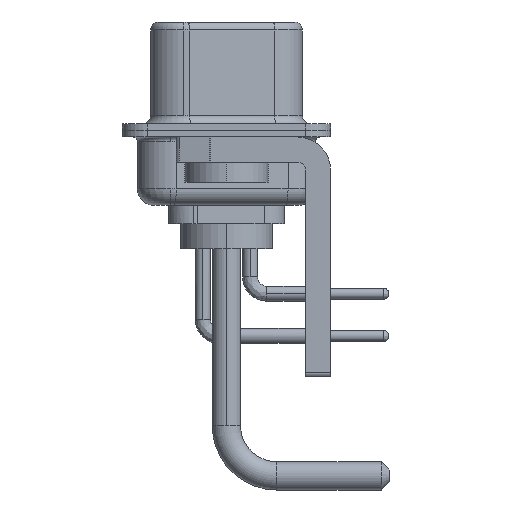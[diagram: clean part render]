
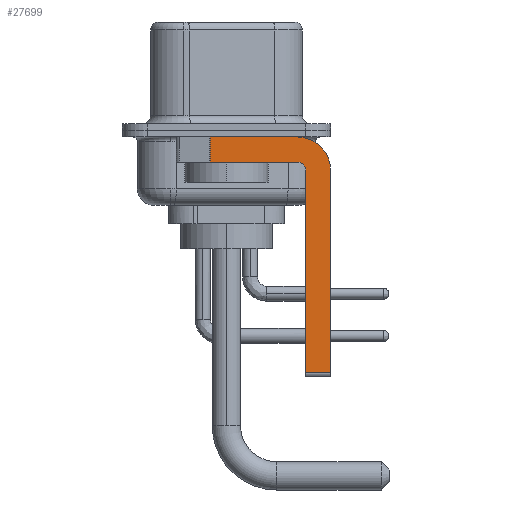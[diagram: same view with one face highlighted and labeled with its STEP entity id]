
A CAD part, left-side view. The second image highlights one B-rep face of the part: STEP entity #27699.
In plain terms, the highlighted planar face has unit normal (-1, 0, 0).
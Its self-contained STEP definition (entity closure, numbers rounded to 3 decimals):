
#1863 = VERTEX_POINT ( 'NONE', #11196 ) ;
#2065 = ORIENTED_EDGE ( 'NONE', *, *, #3485, .T. ) ;
#2196 = VERTEX_POINT ( 'NONE', #10604 ) ;
#3014 = ORIENTED_EDGE ( 'NONE', *, *, #24934, .F. ) ;
#3403 = CARTESIAN_POINT ( 'NONE',  ( -2.9, -6.25, -14.55 ) ) ;
#3485 = EDGE_CURVE ( 'NONE', #23625, #22249, #18943, .T. ) ;
#3623 = EDGE_LOOP ( 'NONE', ( #19286, #19995, #24882, #4847, #15493, #2065, #3014, #16822 ) ) ;
#3652 = CARTESIAN_POINT ( 'NONE',  ( -2.9, -6.25, -2.4 ) ) ;
#3756 = CARTESIAN_POINT ( 'NONE',  ( -2.9, -4.75, -14.8 ) ) ;
#3812 = CARTESIAN_POINT ( 'NONE',  ( -2.9, -4.25, -2.4 ) ) ;
#3895 = DIRECTION ( 'NONE',  ( 0., 1., 0. ) ) ;
#4129 = VECTOR ( 'NONE', #10186, 1000. ) ;
#4389 = CARTESIAN_POINT ( 'NONE',  ( -2.9, -6.25, -2.4 ) ) ;
#4847 = ORIENTED_EDGE ( 'NONE', *, *, #20919, .F. ) ;
#6098 = VECTOR ( 'NONE', #12203, 1000. ) ;
#6399 = CARTESIAN_POINT ( 'NONE',  ( -2.9, 0.978, -1.9 ) ) ;
#6478 = CARTESIAN_POINT ( 'NONE',  ( -2.9, -4.25, -14.55 ) ) ;
#7613 = EDGE_CURVE ( 'NONE', #2196, #16908, #9991, .T. ) ;
#7696 = VECTOR ( 'NONE', #3895, 1000. ) ;
#8020 = DIRECTION ( 'NONE',  ( 0., -1., 0. ) ) ;
#8220 = AXIS2_PLACEMENT_3D ( 'NONE', #10524, #27513, #25687 ) ;
#8608 = CARTESIAN_POINT ( 'NONE',  ( -2.9, -4.25, -1.9 ) ) ;
#9991 = CIRCLE ( 'NONE', #8220, 2. ) ;
#10099 = DIRECTION ( 'NONE',  ( -1., 0., 0. ) ) ;
#10186 = DIRECTION ( 'NONE',  ( 0., 0., 1. ) ) ;
#10524 = CARTESIAN_POINT ( 'NONE',  ( -2.9, -4.25, -2.4 ) ) ;
#10604 = CARTESIAN_POINT ( 'NONE',  ( -2.9, -4.25, -0.4 ) ) ;
#11196 = CARTESIAN_POINT ( 'NONE',  ( -2.9, 0.978, -0.4 ) ) ;
#11369 = EDGE_CURVE ( 'NONE', #1863, #2196, #25261, .T. ) ;
#11616 = AXIS2_PLACEMENT_3D ( 'NONE', #12199, #10099, #18677 ) ;
#12199 = CARTESIAN_POINT ( 'NONE',  ( -2.9, -4.25, -2.4 ) ) ;
#12203 = DIRECTION ( 'NONE',  ( 0., -1., 0. ) ) ;
#12293 = CARTESIAN_POINT ( 'NONE',  ( -2.9, -4.25, -1.9 ) ) ;
#13335 = VECTOR ( 'NONE', #8020, 1000. ) ;
#14727 = DIRECTION ( 'NONE',  ( 1., 0., 0. ) ) ;
#14821 = EDGE_CURVE ( 'NONE', #1863, #21783, #25456, .T. ) ;
#14932 = DIRECTION ( 'NONE',  ( 0., 0., -1. ) ) ;
#15493 = ORIENTED_EDGE ( 'NONE', *, *, #25326, .F. ) ;
#15975 = VERTEX_POINT ( 'NONE', #27261 ) ;
#16437 = CARTESIAN_POINT ( 'NONE',  ( -2.9, 3., -0.4 ) ) ;
#16705 = DIRECTION ( 'NONE',  ( 0., 0., -1. ) ) ;
#16822 = ORIENTED_EDGE ( 'NONE', *, *, #7613, .F. ) ;
#16908 = VERTEX_POINT ( 'NONE', #4389 ) ;
#17076 = VECTOR ( 'NONE', #18926, 1000. ) ;
#17117 = VECTOR ( 'NONE', #14932, 1000. ) ;
#18677 = DIRECTION ( 'NONE',  ( 0., 0., 1. ) ) ;
#18926 = DIRECTION ( 'NONE',  ( 0., 0., -1. ) ) ;
#18943 = LINE ( 'NONE', #6478, #13335 ) ;
#19222 = FACE_OUTER_BOUND ( 'NONE', #3623, .T. ) ;
#19286 = ORIENTED_EDGE ( 'NONE', *, *, #11369, .F. ) ;
#19583 = CARTESIAN_POINT ( 'NONE',  ( -2.9, -4.75, -14.55 ) ) ;
#19995 = ORIENTED_EDGE ( 'NONE', *, *, #14821, .T. ) ;
#20919 = EDGE_CURVE ( 'NONE', #15975, #25299, #26799, .T. ) ;
#21783 = VERTEX_POINT ( 'NONE', #22263 ) ;
#22249 = VERTEX_POINT ( 'NONE', #3403 ) ;
#22263 = CARTESIAN_POINT ( 'NONE',  ( -2.9, 0.978, -1.9 ) ) ;
#22959 = LINE ( 'NONE', #8608, #7696 ) ;
#22964 = LINE ( 'NONE', #3756, #4129 ) ;
#23014 = PLANE ( 'NONE',  #26102 ) ;
#23625 = VERTEX_POINT ( 'NONE', #19583 ) ;
#23970 = EDGE_CURVE ( 'NONE', #25299, #21783, #22959, .T. ) ;
#24882 = ORIENTED_EDGE ( 'NONE', *, *, #23970, .F. ) ;
#24934 = EDGE_CURVE ( 'NONE', #16908, #22249, #25247, .T. ) ;
#25247 = LINE ( 'NONE', #3652, #17076 ) ;
#25261 = LINE ( 'NONE', #16437, #6098 ) ;
#25299 = VERTEX_POINT ( 'NONE', #12293 ) ;
#25326 = EDGE_CURVE ( 'NONE', #23625, #15975, #22964, .T. ) ;
#25456 = LINE ( 'NONE', #6399, #17117 ) ;
#25687 = DIRECTION ( 'NONE',  ( 0., 0., -1. ) ) ;
#26102 = AXIS2_PLACEMENT_3D ( 'NONE', #3812, #14727, #16705 ) ;
#26799 = CIRCLE ( 'NONE', #11616, 0.5 ) ;
#27261 = CARTESIAN_POINT ( 'NONE',  ( -2.9, -4.75, -2.4 ) ) ;
#27513 = DIRECTION ( 'NONE',  ( 1., 0., 0. ) ) ;
#27699 = ADVANCED_FACE ( 'NONE', ( #19222 ), #23014, .F. ) ;
